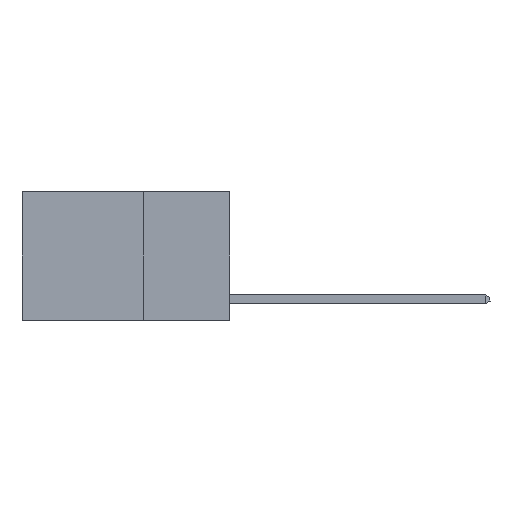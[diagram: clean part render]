
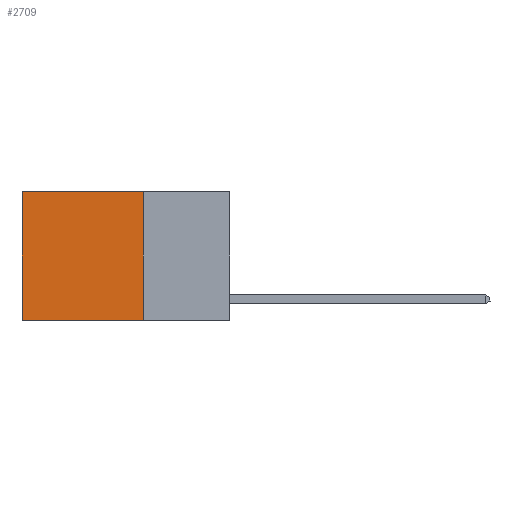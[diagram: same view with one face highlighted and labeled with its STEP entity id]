
A CAD part, left-side view. The second image highlights one B-rep face of the part: STEP entity #2709.
In plain terms, the highlighted planar face has unit normal (-1, 0, 0).
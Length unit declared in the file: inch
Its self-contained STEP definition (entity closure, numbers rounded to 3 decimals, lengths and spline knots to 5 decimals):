
#91 = LINE ( 'NONE', #3400, #4751 ) ;
#134 = CARTESIAN_POINT ( 'NONE',  ( 0.2625, 0.25, 0. ) ) ;
#466 = EDGE_CURVE ( 'NONE', #6844, #4595, #91, .T. ) ;
#617 = CARTESIAN_POINT ( 'NONE',  ( 0.2625, 0.6, 0. ) ) ;
#784 = EDGE_LOOP ( 'NONE', ( #11264, #12198, #5421, #1141 ) ) ;
#1002 = LINE ( 'NONE', #617, #10947 ) ;
#1141 = ORIENTED_EDGE ( 'NONE', *, *, #4087, .T. ) ;
#1566 = DIRECTION ( 'NONE',  ( 0., 1., 0. ) ) ;
#2709 = ADVANCED_FACE ( 'NONE', ( #10851 ), #3046, .F. ) ;
#2852 = LINE ( 'NONE', #4514, #6464 ) ;
#3046 = PLANE ( 'NONE',  #9435 ) ;
#3245 = DIRECTION ( 'NONE',  ( 0., 0., -1. ) ) ;
#3400 = CARTESIAN_POINT ( 'NONE',  ( 0.2625, 0.25, -0.37 ) ) ;
#3613 = CARTESIAN_POINT ( 'NONE',  ( 0.2625, 0.25, -0.37 ) ) ;
#4087 = EDGE_CURVE ( 'NONE', #7418, #7499, #2852, .T. ) ;
#4514 = CARTESIAN_POINT ( 'NONE',  ( 0.2625, 0.25, 0. ) ) ;
#4551 = LINE ( 'NONE', #9967, #11348 ) ;
#4577 = DIRECTION ( 'NONE',  ( 0., 0., -1. ) ) ;
#4595 = VERTEX_POINT ( 'NONE', #9687 ) ;
#4751 = VECTOR ( 'NONE', #1566, 39.37008 ) ;
#4887 = DIRECTION ( 'NONE',  ( 0., 0., -1. ) ) ;
#4920 = EDGE_CURVE ( 'NONE', #7499, #4595, #1002, .T. ) ;
#5421 = ORIENTED_EDGE ( 'NONE', *, *, #7164, .F. ) ;
#6444 = CARTESIAN_POINT ( 'NONE',  ( 0.2625, 0.25, 0. ) ) ;
#6464 = VECTOR ( 'NONE', #8564, 39.37008 ) ;
#6844 = VERTEX_POINT ( 'NONE', #3613 ) ;
#7164 = EDGE_CURVE ( 'NONE', #7418, #6844, #4551, .T. ) ;
#7418 = VERTEX_POINT ( 'NONE', #6444 ) ;
#7499 = VERTEX_POINT ( 'NONE', #10005 ) ;
#8564 = DIRECTION ( 'NONE',  ( 0., 1., 0. ) ) ;
#9435 = AXIS2_PLACEMENT_3D ( 'NONE', #134, #10746, #4887 ) ;
#9687 = CARTESIAN_POINT ( 'NONE',  ( 0.2625, 0.6, -0.37 ) ) ;
#9967 = CARTESIAN_POINT ( 'NONE',  ( 0.2625, 0.25, 0. ) ) ;
#10005 = CARTESIAN_POINT ( 'NONE',  ( 0.2625, 0.6, 0. ) ) ;
#10746 = DIRECTION ( 'NONE',  ( 1., 0., 0. ) ) ;
#10851 = FACE_OUTER_BOUND ( 'NONE', #784, .T. ) ;
#10947 = VECTOR ( 'NONE', #4577, 39.37008 ) ;
#11264 = ORIENTED_EDGE ( 'NONE', *, *, #4920, .T. ) ;
#11348 = VECTOR ( 'NONE', #3245, 39.37008 ) ;
#12198 = ORIENTED_EDGE ( 'NONE', *, *, #466, .F. ) ;
